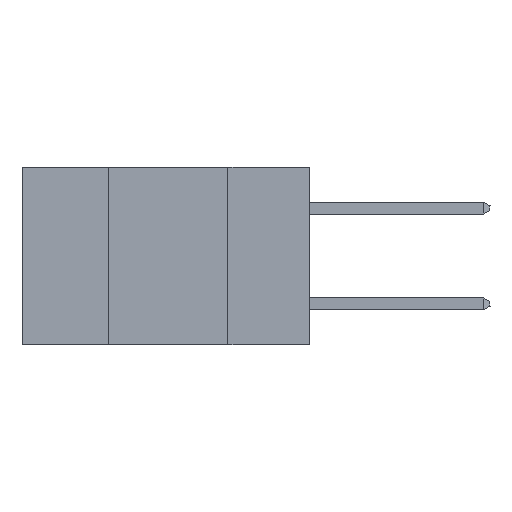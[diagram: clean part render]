
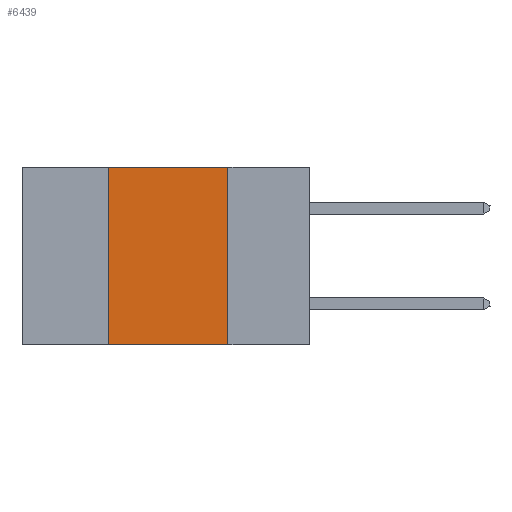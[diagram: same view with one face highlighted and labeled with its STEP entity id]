
A CAD part, left-side view. The second image highlights one B-rep face of the part: STEP entity #6439.
In plain terms, the highlighted planar face has unit normal (-1, 0, 0).
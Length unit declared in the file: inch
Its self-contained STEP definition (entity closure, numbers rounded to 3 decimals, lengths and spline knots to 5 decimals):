
#609 = DIRECTION ( 'NONE',  ( 1., 0., 0. ) ) ;
#821 = ORIENTED_EDGE ( 'NONE', *, *, #10944, .T. ) ;
#857 = VERTEX_POINT ( 'NONE', #6995 ) ;
#996 = EDGE_CURVE ( 'NONE', #1308, #4422, #3881, .T. ) ;
#1308 = VERTEX_POINT ( 'NONE', #9322 ) ;
#2419 = CARTESIAN_POINT ( 'NONE',  ( 0., 0.17, 0. ) ) ;
#2917 = VECTOR ( 'NONE', #9939, 39.37008 ) ;
#3054 = ORIENTED_EDGE ( 'NONE', *, *, #3460, .F. ) ;
#3069 = DIRECTION ( 'NONE',  ( 0., 0., 1. ) ) ;
#3130 = CARTESIAN_POINT ( 'NONE',  ( 0., 0.6, 0. ) ) ;
#3265 = ORIENTED_EDGE ( 'NONE', *, *, #5136, .F. ) ;
#3460 = EDGE_CURVE ( 'NONE', #4422, #4169, #3817, .T. ) ;
#3797 = CARTESIAN_POINT ( 'NONE',  ( 0., 0.6, -0.37 ) ) ;
#3817 = LINE ( 'NONE', #6026, #9419 ) ;
#3881 = LINE ( 'NONE', #8109, #9083 ) ;
#4049 = VECTOR ( 'NONE', #4479, 39.37008 ) ;
#4068 = EDGE_LOOP ( 'NONE', ( #3265, #3054, #10249, #821 ) ) ;
#4169 = VERTEX_POINT ( 'NONE', #2419 ) ;
#4422 = VERTEX_POINT ( 'NONE', #5886 ) ;
#4479 = DIRECTION ( 'NONE',  ( 0., 0., -1. ) ) ;
#5136 = EDGE_CURVE ( 'NONE', #4169, #857, #9775, .T. ) ;
#5886 = CARTESIAN_POINT ( 'NONE',  ( 0., 0.42, 0. ) ) ;
#6026 = CARTESIAN_POINT ( 'NONE',  ( 0., 0.6, 0. ) ) ;
#6372 = AXIS2_PLACEMENT_3D ( 'NONE', #3130, #609, #6526 ) ;
#6439 = ADVANCED_FACE ( 'NONE', ( #10292 ), #8212, .F. ) ;
#6526 = DIRECTION ( 'NONE',  ( 0., 0., -1. ) ) ;
#6992 = CARTESIAN_POINT ( 'NONE',  ( 0., 0.17, 0. ) ) ;
#6995 = CARTESIAN_POINT ( 'NONE',  ( 0., 0.17, -0.37 ) ) ;
#7135 = LINE ( 'NONE', #3797, #2917 ) ;
#8109 = CARTESIAN_POINT ( 'NONE',  ( 0., 0.42, 0. ) ) ;
#8212 = PLANE ( 'NONE',  #6372 ) ;
#8570 = DIRECTION ( 'NONE',  ( 0., -1., 0. ) ) ;
#9083 = VECTOR ( 'NONE', #3069, 39.37008 ) ;
#9322 = CARTESIAN_POINT ( 'NONE',  ( 0., 0.42, -0.37 ) ) ;
#9419 = VECTOR ( 'NONE', #8570, 39.37008 ) ;
#9775 = LINE ( 'NONE', #6992, #4049 ) ;
#9939 = DIRECTION ( 'NONE',  ( 0., -1., 0. ) ) ;
#10249 = ORIENTED_EDGE ( 'NONE', *, *, #996, .F. ) ;
#10292 = FACE_OUTER_BOUND ( 'NONE', #4068, .T. ) ;
#10944 = EDGE_CURVE ( 'NONE', #1308, #857, #7135, .T. ) ;
